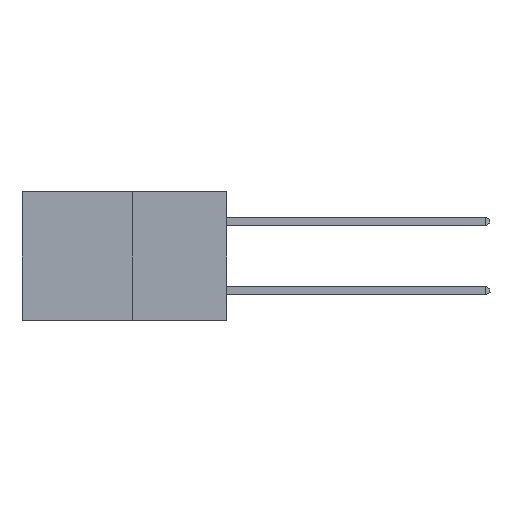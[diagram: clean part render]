
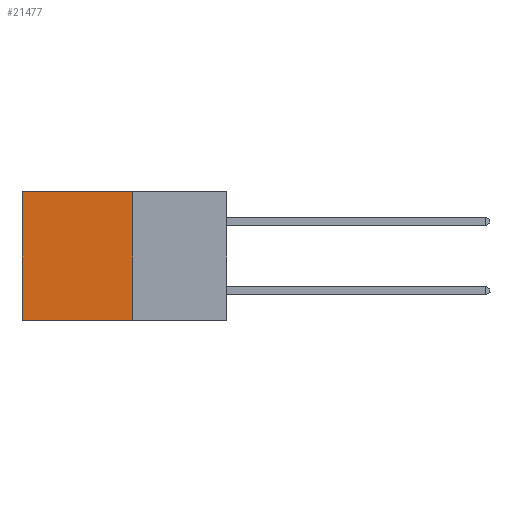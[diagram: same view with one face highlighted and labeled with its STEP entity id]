
A CAD part, left-side view. The second image highlights one B-rep face of the part: STEP entity #21477.
In plain terms, the highlighted planar face has unit normal (-1, 0, 0).
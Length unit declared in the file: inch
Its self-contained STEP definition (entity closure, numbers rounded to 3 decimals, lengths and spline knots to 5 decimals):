
#1599 = CARTESIAN_POINT ( 'NONE',  ( 0.277, 0.59, 0. ) ) ;
#2246 = VECTOR ( 'NONE', #11074, 39.37008 ) ;
#2422 = DIRECTION ( 'NONE',  ( 0., 1., 0. ) ) ;
#2812 = AXIS2_PLACEMENT_3D ( 'NONE', #17166, #6336, #18991 ) ;
#3207 = EDGE_CURVE ( 'NONE', #19679, #5013, #12542, .T. ) ;
#4270 = DIRECTION ( 'NONE',  ( 0., 1., 0. ) ) ;
#4469 = PLANE ( 'NONE',  #2812 ) ;
#4510 = LINE ( 'NONE', #16970, #8821 ) ;
#5013 = VERTEX_POINT ( 'NONE', #18852 ) ;
#5255 = ORIENTED_EDGE ( 'NONE', *, *, #16675, .T. ) ;
#6336 = DIRECTION ( 'NONE',  ( 1., 0., 0. ) ) ;
#6339 = ORIENTED_EDGE ( 'NONE', *, *, #8222, .T. ) ;
#8222 = EDGE_CURVE ( 'NONE', #8260, #17484, #21627, .T. ) ;
#8260 = VERTEX_POINT ( 'NONE', #1599 ) ;
#8821 = VECTOR ( 'NONE', #2422, 39.37008 ) ;
#8894 = VECTOR ( 'NONE', #10714, 39.37008 ) ;
#10592 = CARTESIAN_POINT ( 'NONE',  ( 0.277, 0.27, -0.37 ) ) ;
#10714 = DIRECTION ( 'NONE',  ( 0., 0., -1. ) ) ;
#11074 = DIRECTION ( 'NONE',  ( 0., 0., -1. ) ) ;
#11509 = VECTOR ( 'NONE', #4270, 39.37008 ) ;
#11582 = EDGE_LOOP ( 'NONE', ( #6339, #16537, #21452, #5255 ) ) ;
#12076 = LINE ( 'NONE', #13401, #11509 ) ;
#12542 = LINE ( 'NONE', #10592, #2246 ) ;
#13401 = CARTESIAN_POINT ( 'NONE',  ( 0.277, 0.27, 0. ) ) ;
#13700 = CARTESIAN_POINT ( 'NONE',  ( 0.277, 0.27, 0. ) ) ;
#16537 = ORIENTED_EDGE ( 'NONE', *, *, #19548, .F. ) ;
#16675 = EDGE_CURVE ( 'NONE', #19679, #8260, #12076, .T. ) ;
#16970 = CARTESIAN_POINT ( 'NONE',  ( 0.277, 0.27, -0.37 ) ) ;
#17166 = CARTESIAN_POINT ( 'NONE',  ( 0.277, 0.27, -0.37 ) ) ;
#17484 = VERTEX_POINT ( 'NONE', #18780 ) ;
#18780 = CARTESIAN_POINT ( 'NONE',  ( 0.277, 0.59, -0.37 ) ) ;
#18852 = CARTESIAN_POINT ( 'NONE',  ( 0.277, 0.27, -0.37 ) ) ;
#18991 = DIRECTION ( 'NONE',  ( 0., 0., -1. ) ) ;
#19548 = EDGE_CURVE ( 'NONE', #5013, #17484, #4510, .T. ) ;
#19679 = VERTEX_POINT ( 'NONE', #13700 ) ;
#21452 = ORIENTED_EDGE ( 'NONE', *, *, #3207, .F. ) ;
#21477 = ADVANCED_FACE ( 'NONE', ( #21498 ), #4469, .F. ) ;
#21498 = FACE_OUTER_BOUND ( 'NONE', #11582, .T. ) ;
#21533 = CARTESIAN_POINT ( 'NONE',  ( 0.277, 0.59, -0.37 ) ) ;
#21627 = LINE ( 'NONE', #21533, #8894 ) ;
